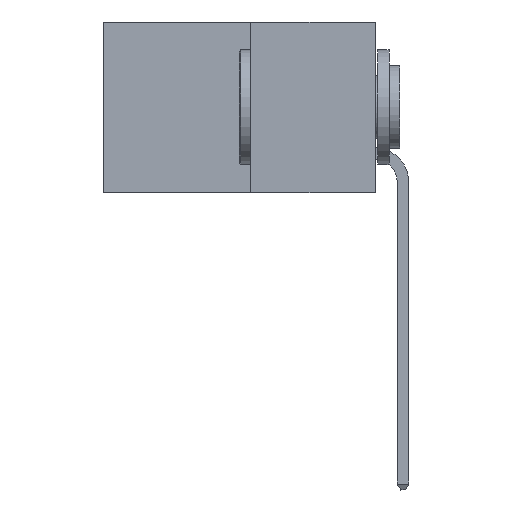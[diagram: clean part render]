
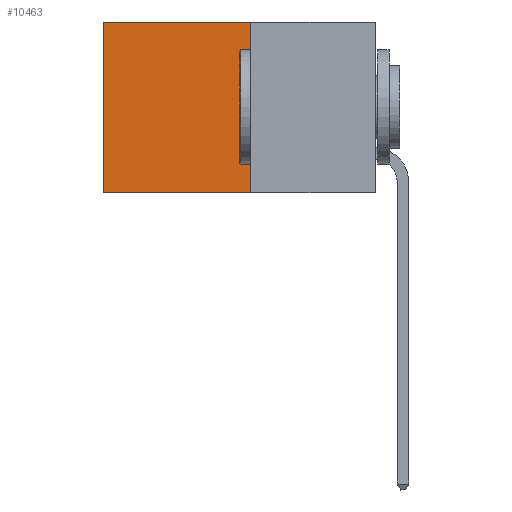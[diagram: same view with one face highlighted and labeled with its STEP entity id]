
A CAD part, left-side view. The second image highlights one B-rep face of the part: STEP entity #10463.
In plain terms, the highlighted planar face has unit normal (-1, 0, 0).
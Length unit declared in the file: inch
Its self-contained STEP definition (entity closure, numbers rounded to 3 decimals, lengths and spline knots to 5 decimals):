
#751 = CARTESIAN_POINT ( 'NONE',  ( 0.277, 0.27, -0.37 ) ) ;
#784 = CARTESIAN_POINT ( 'NONE',  ( 0.277, 0.27, 0. ) ) ;
#857 = VERTEX_POINT ( 'NONE', #17240 ) ;
#893 = EDGE_CURVE ( 'NONE', #14297, #857, #14529, .T. ) ;
#1055 = ORIENTED_EDGE ( 'NONE', *, *, #7487, .F. ) ;
#1131 = LINE ( 'NONE', #784, #5439 ) ;
#1990 = VERTEX_POINT ( 'NONE', #20803 ) ;
#2494 = FACE_OUTER_BOUND ( 'NONE', #18755, .T. ) ;
#2762 = PLANE ( 'NONE',  #5701 ) ;
#4605 = DIRECTION ( 'NONE',  ( 0., 0., -1. ) ) ;
#5439 = VECTOR ( 'NONE', #6321, 39.37008 ) ;
#5701 = AXIS2_PLACEMENT_3D ( 'NONE', #13440, #15235, #4605 ) ;
#6321 = DIRECTION ( 'NONE',  ( 0., 1., 0. ) ) ;
#6767 = ORIENTED_EDGE ( 'NONE', *, *, #8555, .T. ) ;
#7487 = EDGE_CURVE ( 'NONE', #1990, #22716, #19286, .T. ) ;
#8076 = CARTESIAN_POINT ( 'NONE',  ( 0.277, 0.27, -0.37 ) ) ;
#8135 = DIRECTION ( 'NONE',  ( 0., 0., -1. ) ) ;
#8555 = EDGE_CURVE ( 'NONE', #1990, #14297, #1131, .T. ) ;
#9128 = CARTESIAN_POINT ( 'NONE',  ( 0.277, 0.59, -0.37 ) ) ;
#9133 = CARTESIAN_POINT ( 'NONE',  ( 0.277, 0.27, -0.37 ) ) ;
#9990 = VECTOR ( 'NONE', #8135, 39.37008 ) ;
#10463 = ADVANCED_FACE ( 'NONE', ( #2494 ), #2762, .F. ) ;
#13013 = ORIENTED_EDGE ( 'NONE', *, *, #893, .T. ) ;
#13440 = CARTESIAN_POINT ( 'NONE',  ( 0.277, 0.27, -0.37 ) ) ;
#14297 = VERTEX_POINT ( 'NONE', #15699 ) ;
#14529 = LINE ( 'NONE', #9128, #15102 ) ;
#14739 = ORIENTED_EDGE ( 'NONE', *, *, #19050, .F. ) ;
#15102 = VECTOR ( 'NONE', #17464, 39.37008 ) ;
#15235 = DIRECTION ( 'NONE',  ( 1., 0., 0. ) ) ;
#15699 = CARTESIAN_POINT ( 'NONE',  ( 0.277, 0.59, 0. ) ) ;
#17240 = CARTESIAN_POINT ( 'NONE',  ( 0.277, 0.59, -0.37 ) ) ;
#17464 = DIRECTION ( 'NONE',  ( 0., 0., -1. ) ) ;
#17675 = LINE ( 'NONE', #751, #21695 ) ;
#18755 = EDGE_LOOP ( 'NONE', ( #13013, #14739, #1055, #6767 ) ) ;
#19050 = EDGE_CURVE ( 'NONE', #22716, #857, #17675, .T. ) ;
#19286 = LINE ( 'NONE', #8076, #9990 ) ;
#20339 = DIRECTION ( 'NONE',  ( 0., 1., 0. ) ) ;
#20803 = CARTESIAN_POINT ( 'NONE',  ( 0.277, 0.27, 0. ) ) ;
#21695 = VECTOR ( 'NONE', #20339, 39.37008 ) ;
#22716 = VERTEX_POINT ( 'NONE', #9133 ) ;
